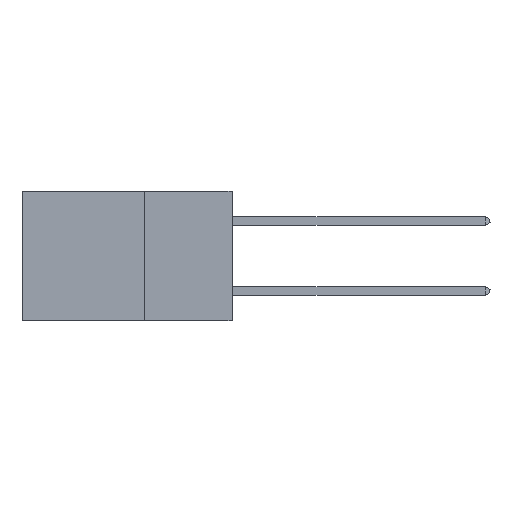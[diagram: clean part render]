
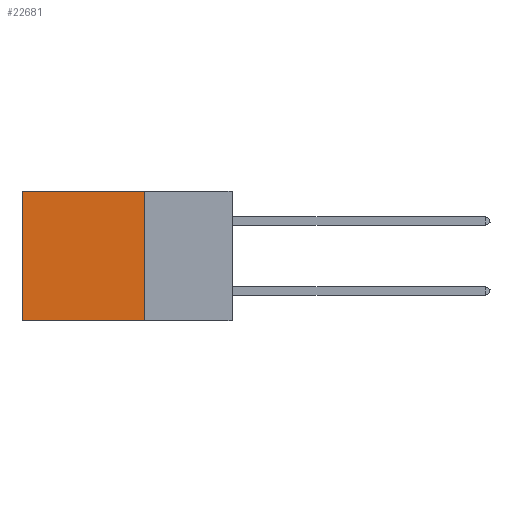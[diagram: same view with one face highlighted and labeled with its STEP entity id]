
A CAD part, left-side view. The second image highlights one B-rep face of the part: STEP entity #22681.
In plain terms, the highlighted planar face has unit normal (-1, 0, 0).
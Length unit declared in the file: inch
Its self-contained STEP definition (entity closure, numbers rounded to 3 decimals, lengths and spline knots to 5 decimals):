
#603 = ORIENTED_EDGE ( 'NONE', *, *, #19410, .T. ) ;
#2552 = EDGE_LOOP ( 'NONE', ( #603, #7757, #3383, #26491 ) ) ;
#2852 = CARTESIAN_POINT ( 'NONE',  ( 0.2875, 0.25, 0. ) ) ;
#3091 = PLANE ( 'NONE',  #3162 ) ;
#3162 = AXIS2_PLACEMENT_3D ( 'NONE', #15527, #25305, #28094 ) ;
#3383 = ORIENTED_EDGE ( 'NONE', *, *, #8565, .F. ) ;
#4709 = CARTESIAN_POINT ( 'NONE',  ( 0.2875, 0.6, 0. ) ) ;
#4909 = CARTESIAN_POINT ( 'NONE',  ( 0.2875, 0.25, 0. ) ) ;
#7757 = ORIENTED_EDGE ( 'NONE', *, *, #19780, .F. ) ;
#8565 = EDGE_CURVE ( 'NONE', #10407, #9519, #15735, .T. ) ;
#9311 = DIRECTION ( 'NONE',  ( 0., 1., 0. ) ) ;
#9519 = VERTEX_POINT ( 'NONE', #26059 ) ;
#10345 = DIRECTION ( 'NONE',  ( 0., 1., 0. ) ) ;
#10407 = VERTEX_POINT ( 'NONE', #2852 ) ;
#11416 = DIRECTION ( 'NONE',  ( 0., 0., -1. ) ) ;
#12314 = VECTOR ( 'NONE', #21908, 39.37008 ) ;
#13101 = LINE ( 'NONE', #31661, #26722 ) ;
#15527 = CARTESIAN_POINT ( 'NONE',  ( 0.2875, 0.25, 0. ) ) ;
#15605 = CARTESIAN_POINT ( 'NONE',  ( 0.2875, 0.6, -0.37 ) ) ;
#15735 = LINE ( 'NONE', #16588, #26593 ) ;
#16588 = CARTESIAN_POINT ( 'NONE',  ( 0.2875, 0.25, 0. ) ) ;
#17095 = CARTESIAN_POINT ( 'NONE',  ( 0.2875, 0.6, 0. ) ) ;
#17988 = FACE_OUTER_BOUND ( 'NONE', #2552, .T. ) ;
#19410 = EDGE_CURVE ( 'NONE', #21191, #24555, #20504, .T. ) ;
#19780 = EDGE_CURVE ( 'NONE', #9519, #24555, #13101, .T. ) ;
#20504 = LINE ( 'NONE', #4709, #12314 ) ;
#20572 = VECTOR ( 'NONE', #10345, 39.37008 ) ;
#21191 = VERTEX_POINT ( 'NONE', #17095 ) ;
#21908 = DIRECTION ( 'NONE',  ( 0., 0., -1. ) ) ;
#22681 = ADVANCED_FACE ( 'NONE', ( #17988 ), #3091, .F. ) ;
#24555 = VERTEX_POINT ( 'NONE', #15605 ) ;
#25305 = DIRECTION ( 'NONE',  ( 1., 0., 0. ) ) ;
#25805 = EDGE_CURVE ( 'NONE', #10407, #21191, #27200, .T. ) ;
#26059 = CARTESIAN_POINT ( 'NONE',  ( 0.2875, 0.25, -0.37 ) ) ;
#26491 = ORIENTED_EDGE ( 'NONE', *, *, #25805, .T. ) ;
#26593 = VECTOR ( 'NONE', #11416, 39.37008 ) ;
#26722 = VECTOR ( 'NONE', #9311, 39.37008 ) ;
#27200 = LINE ( 'NONE', #4909, #20572 ) ;
#28094 = DIRECTION ( 'NONE',  ( 0., 0., -1. ) ) ;
#31661 = CARTESIAN_POINT ( 'NONE',  ( 0.2875, 0.25, -0.37 ) ) ;
